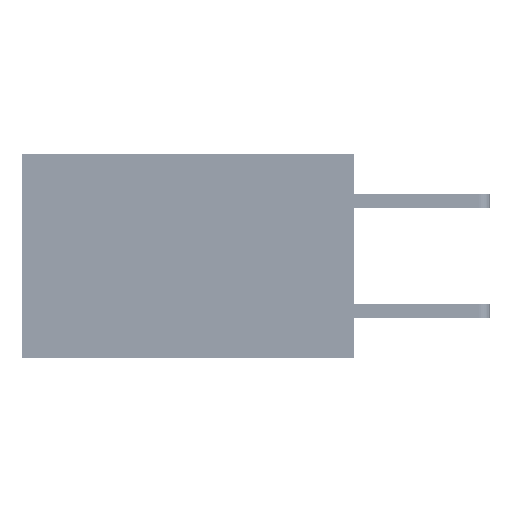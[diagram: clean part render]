
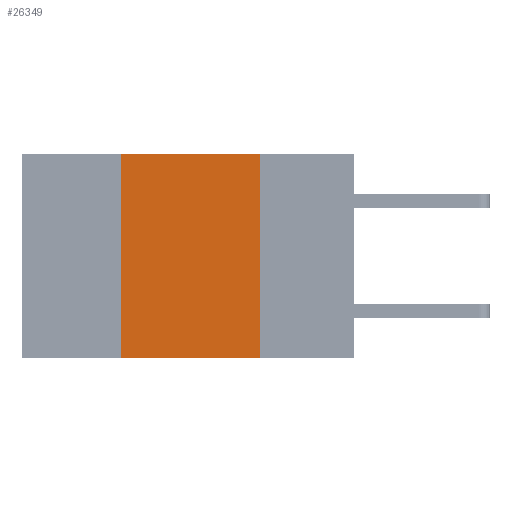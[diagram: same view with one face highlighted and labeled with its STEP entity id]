
A CAD part, left-side view. The second image highlights one B-rep face of the part: STEP entity #26349.
In plain terms, the highlighted planar face has unit normal (-1, 0, 0).
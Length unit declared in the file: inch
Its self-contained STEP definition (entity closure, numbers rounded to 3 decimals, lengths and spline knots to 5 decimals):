
#1443 = DIRECTION ( 'NONE',  ( 0., -1., 0. ) ) ;
#4334 = AXIS2_PLACEMENT_3D ( 'NONE', #11416, #43214, #18912 ) ;
#6884 = DIRECTION ( 'NONE',  ( 0., 0., 1. ) ) ;
#7843 = CARTESIAN_POINT ( 'NONE',  ( 0., 0.42, 0. ) ) ;
#7999 = VECTOR ( 'NONE', #11203, 39.37008 ) ;
#8635 = VERTEX_POINT ( 'NONE', #36450 ) ;
#8876 = ORIENTED_EDGE ( 'NONE', *, *, #51693, .F. ) ;
#8949 = VECTOR ( 'NONE', #6884, 39.37008 ) ;
#9113 = LINE ( 'NONE', #12827, #44775 ) ;
#9524 = DIRECTION ( 'NONE',  ( 0., -1., 0. ) ) ;
#11203 = DIRECTION ( 'NONE',  ( 0., 0., -1. ) ) ;
#11416 = CARTESIAN_POINT ( 'NONE',  ( 0., 0.6, 0. ) ) ;
#12676 = CARTESIAN_POINT ( 'NONE',  ( 0., 0.42, -0.37 ) ) ;
#12827 = CARTESIAN_POINT ( 'NONE',  ( 0., 0.6, -0.37 ) ) ;
#13641 = LINE ( 'NONE', #17692, #48064 ) ;
#14954 = VERTEX_POINT ( 'NONE', #23876 ) ;
#15247 = PLANE ( 'NONE',  #4334 ) ;
#15561 = CARTESIAN_POINT ( 'NONE',  ( 0., 0.17, 0. ) ) ;
#16473 = LINE ( 'NONE', #7843, #8949 ) ;
#17014 = VERTEX_POINT ( 'NONE', #12676 ) ;
#17692 = CARTESIAN_POINT ( 'NONE',  ( 0., 0.6, 0. ) ) ;
#18912 = DIRECTION ( 'NONE',  ( 0., 0., -1. ) ) ;
#20407 = EDGE_CURVE ( 'NONE', #50733, #14954, #31784, .T. ) ;
#23876 = CARTESIAN_POINT ( 'NONE',  ( 0., 0.17, -0.37 ) ) ;
#26349 = ADVANCED_FACE ( 'NONE', ( #48335 ), #15247, .F. ) ;
#29294 = ORIENTED_EDGE ( 'NONE', *, *, #39626, .T. ) ;
#31784 = LINE ( 'NONE', #51395, #7999 ) ;
#35326 = EDGE_CURVE ( 'NONE', #17014, #8635, #16473, .T. ) ;
#36450 = CARTESIAN_POINT ( 'NONE',  ( 0., 0.42, 0. ) ) ;
#39626 = EDGE_CURVE ( 'NONE', #17014, #14954, #9113, .T. ) ;
#39707 = ORIENTED_EDGE ( 'NONE', *, *, #35326, .F. ) ;
#39929 = ORIENTED_EDGE ( 'NONE', *, *, #20407, .F. ) ;
#43214 = DIRECTION ( 'NONE',  ( 1., 0., 0. ) ) ;
#44775 = VECTOR ( 'NONE', #9524, 39.37008 ) ;
#47379 = EDGE_LOOP ( 'NONE', ( #39929, #8876, #39707, #29294 ) ) ;
#48064 = VECTOR ( 'NONE', #1443, 39.37008 ) ;
#48335 = FACE_OUTER_BOUND ( 'NONE', #47379, .T. ) ;
#50733 = VERTEX_POINT ( 'NONE', #15561 ) ;
#51395 = CARTESIAN_POINT ( 'NONE',  ( 0., 0.17, 0. ) ) ;
#51693 = EDGE_CURVE ( 'NONE', #8635, #50733, #13641, .T. ) ;
